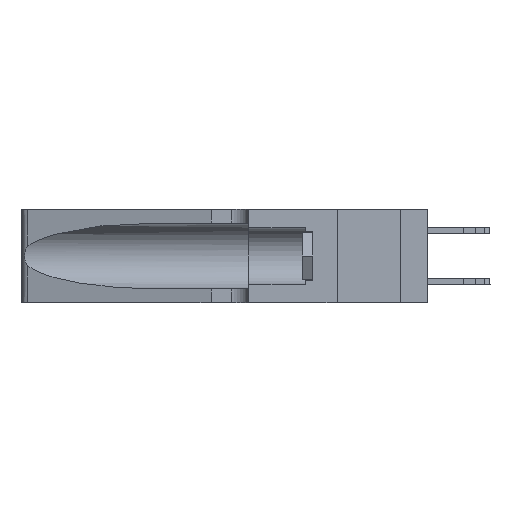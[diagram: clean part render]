
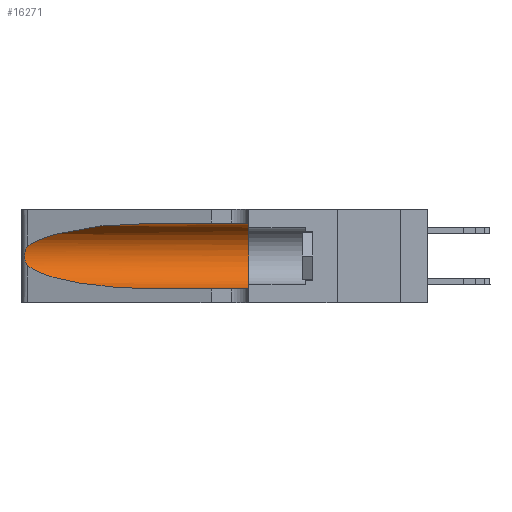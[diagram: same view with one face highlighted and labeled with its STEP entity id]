
A CAD part, left-side view. The second image highlights one B-rep face of the part: STEP entity #16271.
In plain terms, the highlighted cylindrical face has radius 3.308 mm (diameter 6.617 mm), a partial arc.
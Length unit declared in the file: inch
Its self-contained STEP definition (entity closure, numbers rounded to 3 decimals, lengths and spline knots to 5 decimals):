
#52 = ORIENTED_EDGE ( 'NONE', *, *, #7336, .T. ) ;
#226 = VERTEX_POINT ( 'NONE', #11505 ) ;
#486 = DIRECTION ( 'NONE',  ( 0., 1., 0. ) ) ;
#2145 = VECTOR ( 'NONE', #4953, 39.37008 ) ;
#2439 = VERTEX_POINT ( 'NONE', #13239 ) ;
#2782 = EDGE_LOOP ( 'NONE', ( #6959, #52, #16687, #22006, #11274, #24591 ) ) ;
#2864 = CARTESIAN_POINT ( 'NONE',  ( 0.2373, 1.15595, 0.08982 ) ) ;
#3079 = VERTEX_POINT ( 'NONE', #22306 ) ;
#3101 = CARTESIAN_POINT ( 'NONE',  ( 0.1305, 1.61858, 0.185 ) ) ;
#3291 = CARTESIAN_POINT ( 'NONE',  ( 0.1305, 1.61858, 0.05475 ) ) ;
#4155 = CARTESIAN_POINT ( 'NONE',  ( 0.2373, 1.15595, 0.28018 ) ) ;
#4366 = CARTESIAN_POINT ( 'NONE',  ( 0.25789, 1.23486, 0.15765 ) ) ;
#4614 = CARTESIAN_POINT ( 'NONE',  ( 0.25639, 1.23186, 0.15144 ) ) ;
#4953 = DIRECTION ( 'NONE',  ( 0., -1., 0. ) ) ;
#6115 = DIRECTION ( 'NONE',  ( 0., 0., 1. ) ) ;
#6451 = AXIS2_PLACEMENT_3D ( 'NONE', #16647, #486, #6115 ) ;
#6959 = ORIENTED_EDGE ( 'NONE', *, *, #14744, .T. ) ;
#7059 = CIRCLE ( 'NONE', #6451, 0.13025 ) ;
#7336 = EDGE_CURVE ( 'NONE', #31507, #2439, #32891, .T. ) ;
#8795 = LINE ( 'NONE', #15607, #2145 ) ;
#9408 = LINE ( 'NONE', #3291, #13977 ) ;
#10031 = CARTESIAN_POINT ( 'NONE',  ( 0.1305, 0.72297, 0.05475 ) ) ;
#10124 = CARTESIAN_POINT ( 'NONE',  ( 0.26018, 1.23835, 0.19895 ) ) ;
#11274 = ORIENTED_EDGE ( 'NONE', *, *, #34121, .F. ) ;
#11505 = CARTESIAN_POINT ( 'NONE',  ( 0.1305, 0.35, 0.05475 ) ) ;
#11591 = DIRECTION ( 'NONE',  ( 0., 0., -1. ) ) ;
#11609 = CYLINDRICAL_SURFACE ( 'NONE', #12632, 0.13025 ) ;
#11714 = CARTESIAN_POINT ( 'NONE',  ( 0.18966, 0.96281, 0.31525 ) ) ;
#11823 = CARTESIAN_POINT ( 'NONE',  ( 0.1305, 0.35, 0.31525 ) ) ;
#11885 = EDGE_CURVE ( 'NONE', #3079, #12229, #8795, .T. ) ;
#12229 = VERTEX_POINT ( 'NONE', #11823 ) ;
#12304 = CARTESIAN_POINT ( 'NONE',  ( 0.26075, 1.23896, 0.19203 ) ) ;
#12632 = AXIS2_PLACEMENT_3D ( 'NONE', #3101, #25247, #11591 ) ;
#12813 = CARTESIAN_POINT ( 'NONE',  ( 0.26075, 1.23896, 0.178 ) ) ;
#13239 = CARTESIAN_POINT ( 'NONE',  ( 0.25487, 1.22718, 0.14631 ) ) ;
#13977 = VECTOR ( 'NONE', #22324, 39.37008 ) ;
#14153 = FACE_OUTER_BOUND ( 'NONE', #2782, .T. ) ;
#14336 =( BOUNDED_CURVE ( )  B_SPLINE_CURVE ( 3, ( #14421, #11714, #4155, #33158 ),
 .UNSPECIFIED., .F., .F. ) 
 B_SPLINE_CURVE_WITH_KNOTS ( ( 4, 4 ),
 ( 1.5708, 2.84003 ),
 .UNSPECIFIED. ) 
 CURVE ( )  GEOMETRIC_REPRESENTATION_ITEM ( )  RATIONAL_B_SPLINE_CURVE ( ( 1., 0.87, 0.87, 1. ) ) 
 REPRESENTATION_ITEM ( '' )  );
#14421 = CARTESIAN_POINT ( 'NONE',  ( 0.1305, 0.72297, 0.31525 ) ) ;
#14744 = EDGE_CURVE ( 'NONE', #3079, #31507, #14336, .T. ) ;
#15185 = EDGE_CURVE ( 'NONE', #2439, #28778, #32647, .T. ) ;
#15398 = CARTESIAN_POINT ( 'NONE',  ( 0.25856, 1.23593, 0.16098 ) ) ;
#15607 = CARTESIAN_POINT ( 'NONE',  ( 0.1305, 1.61858, 0.31525 ) ) ;
#16202 = CARTESIAN_POINT ( 'NONE',  ( 0.25487, 1.22718, 0.14631 ) ) ;
#16271 = ADVANCED_FACE ( 'NONE', ( #14153 ), #11609, .F. ) ;
#16647 = CARTESIAN_POINT ( 'NONE',  ( 0.1305, 0.35, 0.185 ) ) ;
#16687 = ORIENTED_EDGE ( 'NONE', *, *, #15185, .T. ) ;
#18161 = CARTESIAN_POINT ( 'NONE',  ( 0.25787, 1.23484, 0.2124 ) ) ;
#19745 = CARTESIAN_POINT ( 'NONE',  ( 0.18966, 0.96281, 0.05475 ) ) ;
#20845 = CARTESIAN_POINT ( 'NONE',  ( 0.25854, 1.2359, 0.20912 ) ) ;
#22006 = ORIENTED_EDGE ( 'NONE', *, *, #22142, .T. ) ;
#22142 = EDGE_CURVE ( 'NONE', #28778, #226, #9408, .T. ) ;
#22306 = CARTESIAN_POINT ( 'NONE',  ( 0.1305, 0.72297, 0.31525 ) ) ;
#22324 = DIRECTION ( 'NONE',  ( 0., -1., 0. ) ) ;
#22870 = CARTESIAN_POINT ( 'NONE',  ( 0.1305, 0.72297, 0.05475 ) ) ;
#24591 = ORIENTED_EDGE ( 'NONE', *, *, #11885, .F. ) ;
#25247 = DIRECTION ( 'NONE',  ( 0., -1., 0. ) ) ;
#25847 = CARTESIAN_POINT ( 'NONE',  ( 0.25639, 1.23184, 0.21858 ) ) ;
#26107 = CARTESIAN_POINT ( 'NONE',  ( 0.25487, 1.22718, 0.22369 ) ) ;
#27072 = CARTESIAN_POINT ( 'NONE',  ( 0.25487, 1.22718, 0.22369 ) ) ;
#28288 = CARTESIAN_POINT ( 'NONE',  ( 0.25555, 1.22994, 0.2215 ) ) ;
#28530 = CARTESIAN_POINT ( 'NONE',  ( 0.26017, 1.23833, 0.17102 ) ) ;
#28778 = VERTEX_POINT ( 'NONE', #22870 ) ;
#31184 = CARTESIAN_POINT ( 'NONE',  ( 0.25555, 1.22993, 0.14849 ) ) ;
#31421 = CARTESIAN_POINT ( 'NONE',  ( 0.25487, 1.22718, 0.14631 ) ) ;
#31507 = VERTEX_POINT ( 'NONE', #27072 ) ;
#32647 =( BOUNDED_CURVE ( )  B_SPLINE_CURVE ( 3, ( #16202, #2864, #19745, #10031 ),
 .UNSPECIFIED., .F., .F. ) 
 B_SPLINE_CURVE_WITH_KNOTS ( ( 4, 4 ),
 ( 3.44316, 4.71239 ),
 .UNSPECIFIED. ) 
 CURVE ( )  GEOMETRIC_REPRESENTATION_ITEM ( )  RATIONAL_B_SPLINE_CURVE ( ( 1., 0.87, 0.87, 1. ) ) 
 REPRESENTATION_ITEM ( '' )  );
#32891 = B_SPLINE_CURVE_WITH_KNOTS ( 'NONE', 3,
 ( #26107, #28288, #25847, #18161, #20845, #10124, #12304, #12813, #28530, #15398, #4366, #4614, #31184, #31421 ),
 .UNSPECIFIED., .F., .F.,
 ( 4, 2, 2, 2, 2, 2, 4 ),
 ( 0., 0.00027, 0.00053, 0.00107, 0.0016, 0.00187, 0.00214 ),
 .UNSPECIFIED. ) ;
#33158 = CARTESIAN_POINT ( 'NONE',  ( 0.25487, 1.22718, 0.22369 ) ) ;
#34121 = EDGE_CURVE ( 'NONE', #12229, #226, #7059, .T. ) ;
